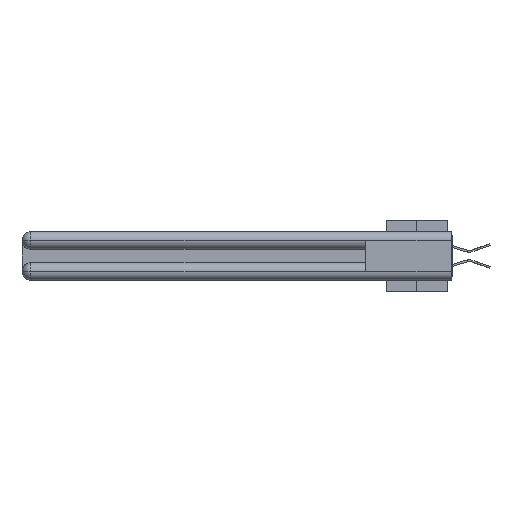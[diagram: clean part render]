
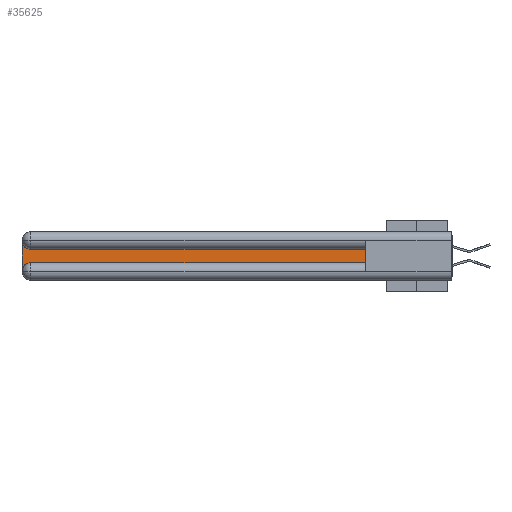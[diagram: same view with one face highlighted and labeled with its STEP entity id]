
A CAD part, left-side view. The second image highlights one B-rep face of the part: STEP entity #35625.
In plain terms, the highlighted planar face has unit normal (-1, 0, 0).
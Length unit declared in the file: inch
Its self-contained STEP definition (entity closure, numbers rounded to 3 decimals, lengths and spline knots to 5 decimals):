
#488 = CARTESIAN_POINT ( 'NONE',  ( 0.075, 0.6, -0.2175 ) ) ;
#1233 = DIRECTION ( 'NONE',  ( 0., 0., 1. ) ) ;
#1964 = AXIS2_PLACEMENT_3D ( 'NONE', #36786, #17874, #20918 ) ;
#2120 = CARTESIAN_POINT ( 'NONE',  ( 0.075, 3., -0.2175 ) ) ;
#3888 = EDGE_CURVE ( 'NONE', #10669, #24966, #36808, .T. ) ;
#4346 = EDGE_CURVE ( 'NONE', #8245, #30935, #5606, .T. ) ;
#4958 = VECTOR ( 'NONE', #5388, 39.37008 ) ;
#5076 = EDGE_CURVE ( 'NONE', #24966, #8245, #6043, .T. ) ;
#5388 = DIRECTION ( 'NONE',  ( 0., 1., 0. ) ) ;
#5606 = CIRCLE ( 'NONE', #15815, 0.06 ) ;
#5987 = CARTESIAN_POINT ( 'NONE',  ( 0.075, 0.6, -0.1225 ) ) ;
#6043 = LINE ( 'NONE', #2120, #21880 ) ;
#6508 = ORIENTED_EDGE ( 'NONE', *, *, #4346, .T. ) ;
#7063 = EDGE_CURVE ( 'NONE', #39620, #10669, #9400, .T. ) ;
#7679 = DIRECTION ( 'NONE',  ( 0., 0., -1. ) ) ;
#8245 = VERTEX_POINT ( 'NONE', #32754 ) ;
#8626 = CARTESIAN_POINT ( 'NONE',  ( 0.075, 0.6, -0.2175 ) ) ;
#8963 = LINE ( 'NONE', #488, #9967 ) ;
#8988 = VERTEX_POINT ( 'NONE', #8626 ) ;
#9400 = LINE ( 'NONE', #14837, #4958 ) ;
#9967 = VECTOR ( 'NONE', #35336, 39.37008 ) ;
#10453 = ORIENTED_EDGE ( 'NONE', *, *, #17896, .T. ) ;
#10669 = VERTEX_POINT ( 'NONE', #12685 ) ;
#10694 = EDGE_CURVE ( 'NONE', #30935, #8988, #8963, .T. ) ;
#12685 = CARTESIAN_POINT ( 'NONE',  ( 0.075, 2.94, -0.1225 ) ) ;
#13063 = CARTESIAN_POINT ( 'NONE',  ( 0.075, 2.94, -0.2175 ) ) ;
#14837 = CARTESIAN_POINT ( 'NONE',  ( 0.075, 0.6, -0.1225 ) ) ;
#15815 = AXIS2_PLACEMENT_3D ( 'NONE', #26951, #39261, #20728 ) ;
#16207 = ORIENTED_EDGE ( 'NONE', *, *, #7063, .T. ) ;
#17385 = PLANE ( 'NONE',  #37117 ) ;
#17613 = EDGE_LOOP ( 'NONE', ( #16207, #25036, #25608, #6508, #31508, #10453 ) ) ;
#17660 = CARTESIAN_POINT ( 'NONE',  ( 0.075, 3., -0.0625 ) ) ;
#17874 = DIRECTION ( 'NONE',  ( 1., 0., 0. ) ) ;
#17896 = EDGE_CURVE ( 'NONE', #8988, #39620, #27200, .T. ) ;
#20081 = CARTESIAN_POINT ( 'NONE',  ( 0.075, 0.6, -0.2175 ) ) ;
#20264 = VECTOR ( 'NONE', #1233, 39.37008 ) ;
#20441 = CARTESIAN_POINT ( 'NONE',  ( 0.075, 3., -0.1225 ) ) ;
#20728 = DIRECTION ( 'NONE',  ( 0., 0., -1. ) ) ;
#20918 = DIRECTION ( 'NONE',  ( 0., 0., -1. ) ) ;
#21880 = VECTOR ( 'NONE', #27456, 39.37008 ) ;
#24966 = VERTEX_POINT ( 'NONE', #17660 ) ;
#25036 = ORIENTED_EDGE ( 'NONE', *, *, #3888, .T. ) ;
#25608 = ORIENTED_EDGE ( 'NONE', *, *, #5076, .T. ) ;
#26951 = CARTESIAN_POINT ( 'NONE',  ( 0.075, 2.94, -0.2775 ) ) ;
#27200 = LINE ( 'NONE', #20081, #20264 ) ;
#27456 = DIRECTION ( 'NONE',  ( 0., 0., -1. ) ) ;
#29231 = FACE_OUTER_BOUND ( 'NONE', #17613, .T. ) ;
#29802 = DIRECTION ( 'NONE',  ( 1., 0., 0. ) ) ;
#30935 = VERTEX_POINT ( 'NONE', #13063 ) ;
#31508 = ORIENTED_EDGE ( 'NONE', *, *, #10694, .T. ) ;
#32754 = CARTESIAN_POINT ( 'NONE',  ( 0.075, 3., -0.2775 ) ) ;
#35336 = DIRECTION ( 'NONE',  ( 0., -1., 0. ) ) ;
#35625 = ADVANCED_FACE ( 'NONE', ( #29231 ), #17385, .F. ) ;
#36786 = CARTESIAN_POINT ( 'NONE',  ( 0.075, 2.94, -0.0625 ) ) ;
#36808 = CIRCLE ( 'NONE', #1964, 0.06 ) ;
#37117 = AXIS2_PLACEMENT_3D ( 'NONE', #20441, #29802, #7679 ) ;
#39261 = DIRECTION ( 'NONE',  ( 1., 0., 0. ) ) ;
#39620 = VERTEX_POINT ( 'NONE', #5987 ) ;
